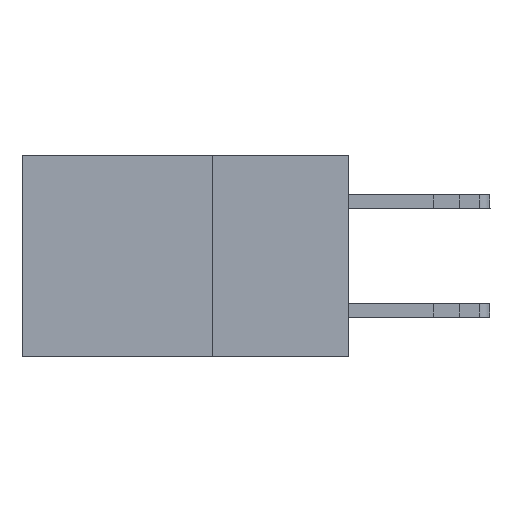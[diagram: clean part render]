
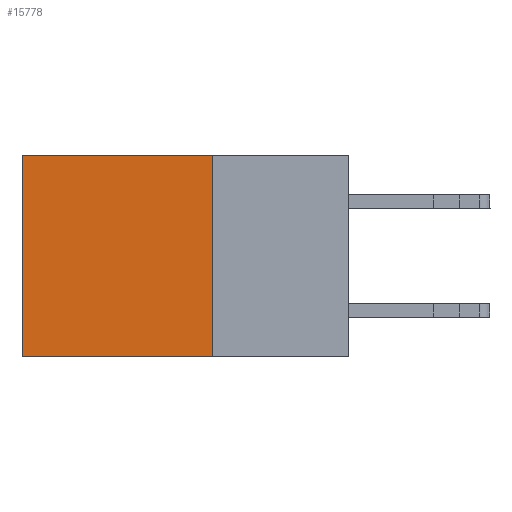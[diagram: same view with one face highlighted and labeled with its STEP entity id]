
A CAD part, left-side view. The second image highlights one B-rep face of the part: STEP entity #15778.
In plain terms, the highlighted planar face has unit normal (-1, 0, 0).
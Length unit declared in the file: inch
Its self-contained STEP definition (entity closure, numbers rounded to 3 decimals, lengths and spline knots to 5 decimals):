
#208 = CARTESIAN_POINT ( 'NONE',  ( 0.2615, 0.25, -0.37 ) ) ;
#244 = ORIENTED_EDGE ( 'NONE', *, *, #15099, .T. ) ;
#753 = ORIENTED_EDGE ( 'NONE', *, *, #1729, .F. ) ;
#1511 = VERTEX_POINT ( 'NONE', #9791 ) ;
#1729 = EDGE_CURVE ( 'NONE', #6807, #2250, #13785, .T. ) ;
#2097 = CARTESIAN_POINT ( 'NONE',  ( 0.2615, 0.25, -0.37 ) ) ;
#2250 = VERTEX_POINT ( 'NONE', #7225 ) ;
#2391 = CARTESIAN_POINT ( 'NONE',  ( 0.2615, 0.25, -0.37 ) ) ;
#2712 = FACE_OUTER_BOUND ( 'NONE', #10343, .T. ) ;
#3223 = VECTOR ( 'NONE', #3355, 39.37008 ) ;
#3355 = DIRECTION ( 'NONE',  ( 0., 0., -1. ) ) ;
#3580 = DIRECTION ( 'NONE',  ( 0., 1., 0. ) ) ;
#3814 = ORIENTED_EDGE ( 'NONE', *, *, #13164, .F. ) ;
#5051 = CARTESIAN_POINT ( 'NONE',  ( 0.2615, 0.25, 0. ) ) ;
#5592 = VECTOR ( 'NONE', #3580, 39.37008 ) ;
#5872 = VECTOR ( 'NONE', #15371, 39.37008 ) ;
#5954 = CARTESIAN_POINT ( 'NONE',  ( 0.2615, 0.6, -0.37 ) ) ;
#6099 = EDGE_CURVE ( 'NONE', #16039, #1511, #8655, .T. ) ;
#6807 = VERTEX_POINT ( 'NONE', #14790 ) ;
#6952 = ORIENTED_EDGE ( 'NONE', *, *, #6099, .T. ) ;
#7182 = VECTOR ( 'NONE', #12787, 39.37008 ) ;
#7225 = CARTESIAN_POINT ( 'NONE',  ( 0.2615, 0.25, -0.37 ) ) ;
#7401 = CARTESIAN_POINT ( 'NONE',  ( 0.2615, 0.6, 0. ) ) ;
#7530 = LINE ( 'NONE', #5051, #5592 ) ;
#8655 = LINE ( 'NONE', #5954, #3223 ) ;
#9791 = CARTESIAN_POINT ( 'NONE',  ( 0.2615, 0.6, -0.37 ) ) ;
#10343 = EDGE_LOOP ( 'NONE', ( #6952, #3814, #753, #244 ) ) ;
#11368 = LINE ( 'NONE', #2391, #7182 ) ;
#12787 = DIRECTION ( 'NONE',  ( 0., 1., 0. ) ) ;
#12925 = DIRECTION ( 'NONE',  ( 0., 0., -1. ) ) ;
#13164 = EDGE_CURVE ( 'NONE', #2250, #1511, #11368, .T. ) ;
#13785 = LINE ( 'NONE', #2097, #5872 ) ;
#14302 = PLANE ( 'NONE',  #15626 ) ;
#14790 = CARTESIAN_POINT ( 'NONE',  ( 0.2615, 0.25, 0. ) ) ;
#15099 = EDGE_CURVE ( 'NONE', #6807, #16039, #7530, .T. ) ;
#15371 = DIRECTION ( 'NONE',  ( 0., 0., -1. ) ) ;
#15626 = AXIS2_PLACEMENT_3D ( 'NONE', #208, #16772, #12925 ) ;
#15778 = ADVANCED_FACE ( 'NONE', ( #2712 ), #14302, .F. ) ;
#16039 = VERTEX_POINT ( 'NONE', #7401 ) ;
#16772 = DIRECTION ( 'NONE',  ( 1., 0., 0. ) ) ;
